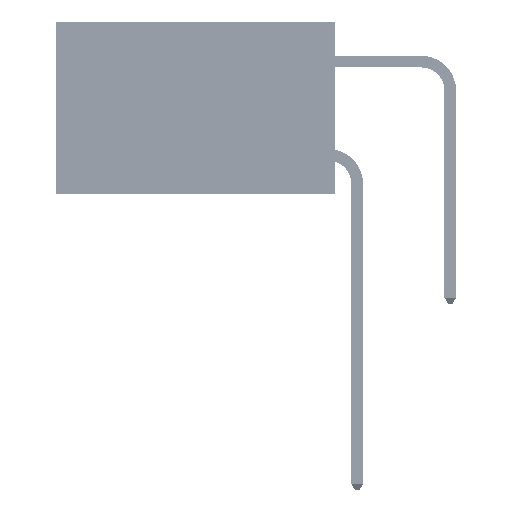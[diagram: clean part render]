
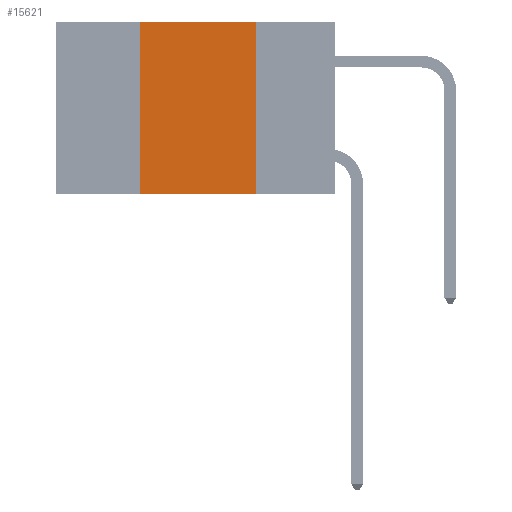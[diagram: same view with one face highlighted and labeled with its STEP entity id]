
A CAD part, left-side view. The second image highlights one B-rep face of the part: STEP entity #15621.
In plain terms, the highlighted planar face has unit normal (-1, 0, 0).
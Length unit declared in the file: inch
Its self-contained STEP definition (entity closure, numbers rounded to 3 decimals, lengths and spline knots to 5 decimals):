
#2952 = PLANE ( 'NONE',  #15532 ) ;
#5550 = ORIENTED_EDGE ( 'NONE', *, *, #52525, .F. ) ;
#7305 = VECTOR ( 'NONE', #17210, 39.37008 ) ;
#9200 = ORIENTED_EDGE ( 'NONE', *, *, #13394, .T. ) ;
#9403 = CARTESIAN_POINT ( 'NONE',  ( 0., 0.6, -0.37 ) ) ;
#9634 = CARTESIAN_POINT ( 'NONE',  ( 0., 0.42, 0. ) ) ;
#11589 = DIRECTION ( 'NONE',  ( 0., 0., -1. ) ) ;
#13394 = EDGE_CURVE ( 'NONE', #30243, #36613, #32004, .T. ) ;
#15413 = CARTESIAN_POINT ( 'NONE',  ( 0., 0.6, 0. ) ) ;
#15532 = AXIS2_PLACEMENT_3D ( 'NONE', #15413, #19638, #11589 ) ;
#15621 = ADVANCED_FACE ( 'NONE', ( #33877 ), #2952, .F. ) ;
#15668 = CARTESIAN_POINT ( 'NONE',  ( 0., 0.42, -0.37 ) ) ;
#16472 = ORIENTED_EDGE ( 'NONE', *, *, #50754, .F. ) ;
#17210 = DIRECTION ( 'NONE',  ( 0., 0., 1. ) ) ;
#18356 = VERTEX_POINT ( 'NONE', #9634 ) ;
#19638 = DIRECTION ( 'NONE',  ( 1., 0., 0. ) ) ;
#20023 = CARTESIAN_POINT ( 'NONE',  ( 0., 0.6, 0. ) ) ;
#21076 = CARTESIAN_POINT ( 'NONE',  ( 0., 0.42, 0. ) ) ;
#22394 = LINE ( 'NONE', #21076, #7305 ) ;
#23689 = ORIENTED_EDGE ( 'NONE', *, *, #51172, .F. ) ;
#27536 = VECTOR ( 'NONE', #45339, 39.37008 ) ;
#30243 = VERTEX_POINT ( 'NONE', #15668 ) ;
#31920 = VECTOR ( 'NONE', #49423, 39.37008 ) ;
#32004 = LINE ( 'NONE', #9403, #52922 ) ;
#32706 = CARTESIAN_POINT ( 'NONE',  ( 0., 0.17, 0. ) ) ;
#33877 = FACE_OUTER_BOUND ( 'NONE', #36958, .T. ) ;
#34740 = CARTESIAN_POINT ( 'NONE',  ( 0., 0.17, -0.37 ) ) ;
#35182 = DIRECTION ( 'NONE',  ( 0., -1., 0. ) ) ;
#36491 = LINE ( 'NONE', #20023, #31920 ) ;
#36613 = VERTEX_POINT ( 'NONE', #34740 ) ;
#36958 = EDGE_LOOP ( 'NONE', ( #23689, #5550, #16472, #9200 ) ) ;
#38653 = LINE ( 'NONE', #32706, #27536 ) ;
#40702 = CARTESIAN_POINT ( 'NONE',  ( 0., 0.17, 0. ) ) ;
#44932 = VERTEX_POINT ( 'NONE', #40702 ) ;
#45339 = DIRECTION ( 'NONE',  ( 0., 0., -1. ) ) ;
#49423 = DIRECTION ( 'NONE',  ( 0., -1., 0. ) ) ;
#50754 = EDGE_CURVE ( 'NONE', #30243, #18356, #22394, .T. ) ;
#51172 = EDGE_CURVE ( 'NONE', #44932, #36613, #38653, .T. ) ;
#52525 = EDGE_CURVE ( 'NONE', #18356, #44932, #36491, .T. ) ;
#52922 = VECTOR ( 'NONE', #35182, 39.37008 ) ;
